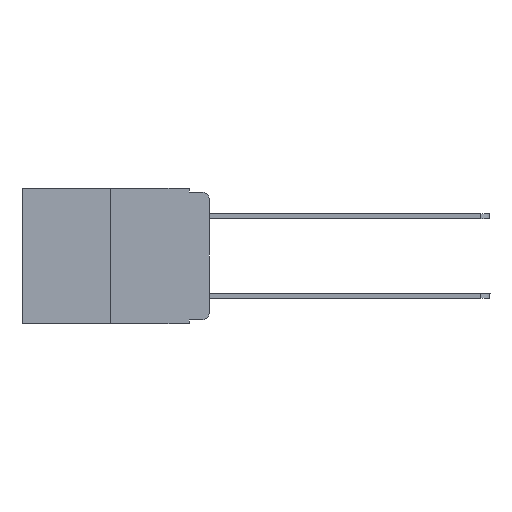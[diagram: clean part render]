
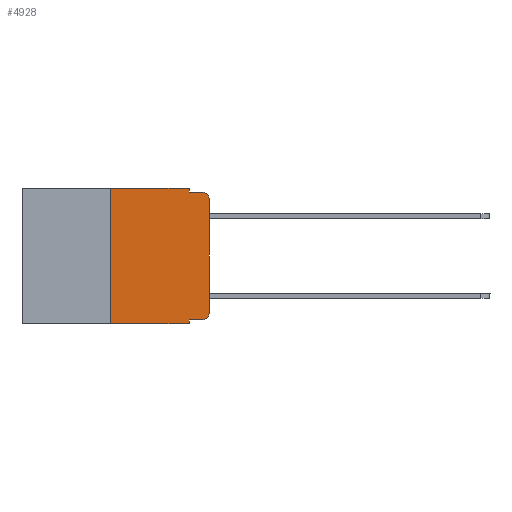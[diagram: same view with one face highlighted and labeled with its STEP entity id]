
A CAD part, left-side view. The second image highlights one B-rep face of the part: STEP entity #4928.
In plain terms, the highlighted planar face has unit normal (-1, 0, 0).
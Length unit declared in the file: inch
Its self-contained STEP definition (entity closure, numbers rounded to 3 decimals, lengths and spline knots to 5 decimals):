
#7 = VERTEX_POINT ( 'NONE', #8126 ) ;
#199 = FACE_OUTER_BOUND ( 'NONE', #5251, .T. ) ;
#215 = DIRECTION ( 'NONE',  ( 0., 0., -1. ) ) ;
#271 = LINE ( 'NONE', #5037, #6129 ) ;
#338 = CARTESIAN_POINT ( 'NONE',  ( 0., 0.473, 0. ) ) ;
#578 = AXIS2_PLACEMENT_3D ( 'NONE', #2413, #6486, #6370 ) ;
#700 = LINE ( 'NONE', #8900, #9942 ) ;
#1025 = CARTESIAN_POINT ( 'NONE',  ( 0., 0., -0.03 ) ) ;
#1537 = ORIENTED_EDGE ( 'NONE', *, *, #7160, .T. ) ;
#1735 = DIRECTION ( 'NONE',  ( 0., 0., 1. ) ) ;
#1851 = CARTESIAN_POINT ( 'NONE',  ( 0., 0.051, -0.01 ) ) ;
#2324 = CIRCLE ( 'NONE', #3963, 0.02 ) ;
#2325 = CARTESIAN_POINT ( 'NONE',  ( 0., 0.051, -0.01 ) ) ;
#2413 = CARTESIAN_POINT ( 'NONE',  ( 0., 0.02, -0.03 ) ) ;
#2439 = EDGE_CURVE ( 'NONE', #7, #3036, #2324, .T. ) ;
#2529 = EDGE_CURVE ( 'NONE', #8761, #8636, #11654, .T. ) ;
#2558 = CARTESIAN_POINT ( 'NONE',  ( 0., 0.051, 0. ) ) ;
#2614 = EDGE_CURVE ( 'NONE', #8024, #5502, #700, .T. ) ;
#2837 = ORIENTED_EDGE ( 'NONE', *, *, #2439, .T. ) ;
#3031 = VERTEX_POINT ( 'NONE', #10644 ) ;
#3036 = VERTEX_POINT ( 'NONE', #12625 ) ;
#3410 = VECTOR ( 'NONE', #8880, 39.37008 ) ;
#3546 = VECTOR ( 'NONE', #12005, 39.37008 ) ;
#3804 = VECTOR ( 'NONE', #8846, 39.37008 ) ;
#3880 = ORIENTED_EDGE ( 'NONE', *, *, #12410, .T. ) ;
#3963 = AXIS2_PLACEMENT_3D ( 'NONE', #6163, #4130, #8189 ) ;
#3997 = CARTESIAN_POINT ( 'NONE',  ( 0., 0.051, 0. ) ) ;
#4060 = CARTESIAN_POINT ( 'NONE',  ( 0., 0., 0. ) ) ;
#4061 = LINE ( 'NONE', #3997, #5478 ) ;
#4073 = ORIENTED_EDGE ( 'NONE', *, *, #2614, .F. ) ;
#4130 = DIRECTION ( 'NONE',  ( -1., 0., 0. ) ) ;
#4166 = PLANE ( 'NONE',  #10401 ) ;
#4520 = VERTEX_POINT ( 'NONE', #7273 ) ;
#4596 = ORIENTED_EDGE ( 'NONE', *, *, #8662, .F. ) ;
#4928 = ADVANCED_FACE ( 'NONE', ( #199 ), #4166, .F. ) ;
#5037 = CARTESIAN_POINT ( 'NONE',  ( 0., 0.473, 0. ) ) ;
#5170 = ORIENTED_EDGE ( 'NONE', *, *, #9444, .T. ) ;
#5251 = EDGE_LOOP ( 'NONE', ( #1537, #11999, #12102, #7831, #12265, #4073, #5170, #4596, #3880, #2837 ) ) ;
#5478 = VECTOR ( 'NONE', #215, 39.37008 ) ;
#5502 = VERTEX_POINT ( 'NONE', #8572 ) ;
#5661 = CARTESIAN_POINT ( 'NONE',  ( 0., 0.051, -0.333 ) ) ;
#5781 = LINE ( 'NONE', #10786, #3804 ) ;
#6129 = VECTOR ( 'NONE', #9078, 39.37008 ) ;
#6163 = CARTESIAN_POINT ( 'NONE',  ( 0., 0.02, -0.313 ) ) ;
#6370 = DIRECTION ( 'NONE',  ( 0., 0., -1. ) ) ;
#6486 = DIRECTION ( 'NONE',  ( -1., 0., 0. ) ) ;
#6623 = LINE ( 'NONE', #5661, #12776 ) ;
#7160 = EDGE_CURVE ( 'NONE', #3036, #8761, #7985, .T. ) ;
#7272 = CARTESIAN_POINT ( 'NONE',  ( 0., 0.02, -0.01 ) ) ;
#7273 = CARTESIAN_POINT ( 'NONE',  ( 0., 0.051, -0.333 ) ) ;
#7831 = ORIENTED_EDGE ( 'NONE', *, *, #12435, .F. ) ;
#7985 = LINE ( 'NONE', #4060, #3546 ) ;
#8024 = VERTEX_POINT ( 'NONE', #11891 ) ;
#8026 = VERTEX_POINT ( 'NONE', #10782 ) ;
#8048 = VECTOR ( 'NONE', #10472, 39.37008 ) ;
#8126 = CARTESIAN_POINT ( 'NONE',  ( 0., 0.02, -0.333 ) ) ;
#8159 = DIRECTION ( 'NONE',  ( 1., 0., 0. ) ) ;
#8189 = DIRECTION ( 'NONE',  ( 0., 0., -1. ) ) ;
#8572 = CARTESIAN_POINT ( 'NONE',  ( 0., 0.25, 0. ) ) ;
#8636 = VERTEX_POINT ( 'NONE', #7272 ) ;
#8662 = EDGE_CURVE ( 'NONE', #4520, #3031, #4061, .T. ) ;
#8752 = VERTEX_POINT ( 'NONE', #2325 ) ;
#8761 = VERTEX_POINT ( 'NONE', #1025 ) ;
#8846 = DIRECTION ( 'NONE',  ( 0., -1., 0. ) ) ;
#8880 = DIRECTION ( 'NONE',  ( 0., -1., 0. ) ) ;
#8900 = CARTESIAN_POINT ( 'NONE',  ( 0., 0.25, 0. ) ) ;
#9078 = DIRECTION ( 'NONE',  ( 0., -1., 0. ) ) ;
#9444 = EDGE_CURVE ( 'NONE', #8024, #3031, #5781, .T. ) ;
#9851 = LINE ( 'NONE', #1851, #3410 ) ;
#9942 = VECTOR ( 'NONE', #1735, 39.37008 ) ;
#10391 = EDGE_CURVE ( 'NONE', #8752, #8636, #9851, .T. ) ;
#10401 = AXIS2_PLACEMENT_3D ( 'NONE', #338, #8159, #12047 ) ;
#10472 = DIRECTION ( 'NONE',  ( 0., 0., -1. ) ) ;
#10525 = EDGE_CURVE ( 'NONE', #5502, #8026, #271, .T. ) ;
#10644 = CARTESIAN_POINT ( 'NONE',  ( 0., 0.051, -0.343 ) ) ;
#10782 = CARTESIAN_POINT ( 'NONE',  ( 0., 0.051, 0. ) ) ;
#10786 = CARTESIAN_POINT ( 'NONE',  ( 0., 0.473, -0.343 ) ) ;
#11456 = LINE ( 'NONE', #2558, #8048 ) ;
#11520 = DIRECTION ( 'NONE',  ( 0., -1., 0. ) ) ;
#11654 = CIRCLE ( 'NONE', #578, 0.02 ) ;
#11891 = CARTESIAN_POINT ( 'NONE',  ( 0., 0.25, -0.343 ) ) ;
#11999 = ORIENTED_EDGE ( 'NONE', *, *, #2529, .T. ) ;
#12005 = DIRECTION ( 'NONE',  ( 0., 0., 1. ) ) ;
#12047 = DIRECTION ( 'NONE',  ( 0., 0., -1. ) ) ;
#12102 = ORIENTED_EDGE ( 'NONE', *, *, #10391, .F. ) ;
#12265 = ORIENTED_EDGE ( 'NONE', *, *, #10525, .F. ) ;
#12410 = EDGE_CURVE ( 'NONE', #4520, #7, #6623, .T. ) ;
#12435 = EDGE_CURVE ( 'NONE', #8026, #8752, #11456, .T. ) ;
#12625 = CARTESIAN_POINT ( 'NONE',  ( 0., 0., -0.313 ) ) ;
#12776 = VECTOR ( 'NONE', #11520, 39.37008 ) ;
